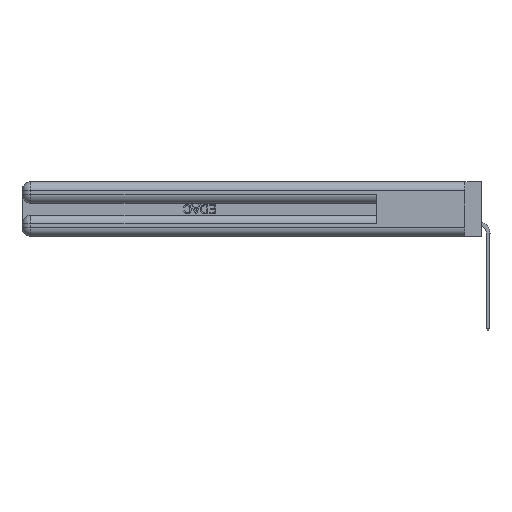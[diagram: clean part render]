
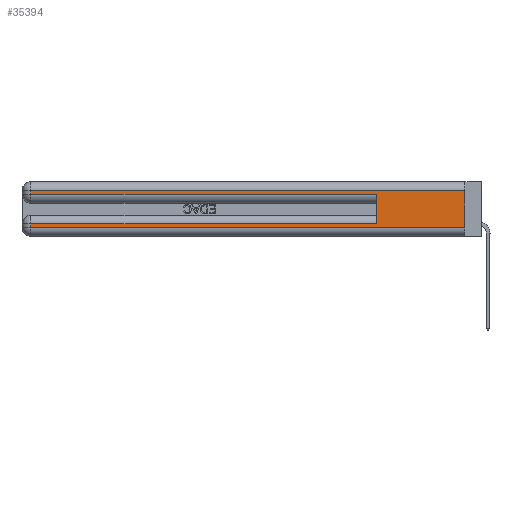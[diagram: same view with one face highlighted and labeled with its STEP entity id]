
A CAD part, left-side view. The second image highlights one B-rep face of the part: STEP entity #35394.
In plain terms, the highlighted planar face has unit normal (-1, 0, 0).
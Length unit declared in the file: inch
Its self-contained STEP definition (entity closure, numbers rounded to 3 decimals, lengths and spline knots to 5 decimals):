
#457 = CARTESIAN_POINT ( 'NONE',  ( 0., 2.94, 0.285 ) ) ;
#775 = EDGE_CURVE ( 'NONE', #44363, #33501, #40268, .T. ) ;
#856 = ORIENTED_EDGE ( 'NONE', *, *, #20694, .T. ) ;
#1387 = CARTESIAN_POINT ( 'NONE',  ( 0., 2.94, 0.37 ) ) ;
#3779 = EDGE_CURVE ( 'NONE', #34875, #40373, #24281, .T. ) ;
#3795 = VECTOR ( 'NONE', #15402, 39.37008 ) ;
#4311 = CARTESIAN_POINT ( 'NONE',  ( 0., 0.6, 0.145 ) ) ;
#4774 = VECTOR ( 'NONE', #35210, 39.37008 ) ;
#5771 = DIRECTION ( 'NONE',  ( 0., -1., 0. ) ) ;
#5900 = CARTESIAN_POINT ( 'NONE',  ( 0., 0., 0.31 ) ) ;
#5971 = DIRECTION ( 'NONE',  ( 0., 0., -1. ) ) ;
#6256 = LINE ( 'NONE', #1387, #13732 ) ;
#6915 = EDGE_CURVE ( 'NONE', #35294, #33501, #15475, .T. ) ;
#9923 = CARTESIAN_POINT ( 'NONE',  ( 0., 2.94, 0.37 ) ) ;
#11583 = ORIENTED_EDGE ( 'NONE', *, *, #41919, .T. ) ;
#12135 = CARTESIAN_POINT ( 'NONE',  ( 0., 0., 0.285 ) ) ;
#13319 = DIRECTION ( 'NONE',  ( 0., 0., -1. ) ) ;
#13518 = EDGE_CURVE ( 'NONE', #40814, #44363, #6256, .T. ) ;
#13732 = VECTOR ( 'NONE', #28822, 39.37008 ) ;
#14787 = DIRECTION ( 'NONE',  ( 0., 0., -1. ) ) ;
#15099 = AXIS2_PLACEMENT_3D ( 'NONE', #43406, #29791, #5971 ) ;
#15130 = VECTOR ( 'NONE', #27407, 39.37008 ) ;
#15402 = DIRECTION ( 'NONE',  ( 0., -1., 0. ) ) ;
#15475 = LINE ( 'NONE', #4311, #4774 ) ;
#16204 = DIRECTION ( 'NONE',  ( 0., 1., 0. ) ) ;
#17505 = CARTESIAN_POINT ( 'NONE',  ( 0., 0., 0.085 ) ) ;
#19222 = FACE_OUTER_BOUND ( 'NONE', #30261, .T. ) ;
#19394 = LINE ( 'NONE', #17505, #15130 ) ;
#20512 = LINE ( 'NONE', #22964, #35559 ) ;
#20694 = EDGE_CURVE ( 'NONE', #34875, #40814, #29694, .T. ) ;
#21058 = CARTESIAN_POINT ( 'NONE',  ( 0., 0., 0.37 ) ) ;
#22111 = VECTOR ( 'NONE', #14787, 39.37008 ) ;
#22132 = LINE ( 'NONE', #9923, #26971 ) ;
#22964 = CARTESIAN_POINT ( 'NONE',  ( 0., 0., 0.06 ) ) ;
#24281 = LINE ( 'NONE', #21058, #22111 ) ;
#26465 = PLANE ( 'NONE',  #15099 ) ;
#26871 = ORIENTED_EDGE ( 'NONE', *, *, #775, .T. ) ;
#26971 = VECTOR ( 'NONE', #13319, 39.37008 ) ;
#27209 = CARTESIAN_POINT ( 'NONE',  ( 0., 0., 0.06 ) ) ;
#27407 = DIRECTION ( 'NONE',  ( 0., 1., 0. ) ) ;
#27806 = CARTESIAN_POINT ( 'NONE',  ( 0., 2.94, 0.085 ) ) ;
#28135 = VERTEX_POINT ( 'NONE', #27806 ) ;
#28822 = DIRECTION ( 'NONE',  ( 0., 0., -1. ) ) ;
#29315 = CARTESIAN_POINT ( 'NONE',  ( 0., 0., 0.31 ) ) ;
#29694 = LINE ( 'NONE', #5900, #34015 ) ;
#29716 = ORIENTED_EDGE ( 'NONE', *, *, #13518, .T. ) ;
#29791 = DIRECTION ( 'NONE',  ( 1., 0., 0. ) ) ;
#30261 = EDGE_LOOP ( 'NONE', ( #31614, #856, #29716, #26871, #39343, #40999, #11583, #32832 ) ) ;
#31614 = ORIENTED_EDGE ( 'NONE', *, *, #3779, .F. ) ;
#32832 = ORIENTED_EDGE ( 'NONE', *, *, #38927, .T. ) ;
#33501 = VERTEX_POINT ( 'NONE', #44139 ) ;
#33591 = CARTESIAN_POINT ( 'NONE',  ( 0., 2.94, 0.31 ) ) ;
#34015 = VECTOR ( 'NONE', #16204, 39.37008 ) ;
#34579 = EDGE_CURVE ( 'NONE', #35294, #28135, #19394, .T. ) ;
#34875 = VERTEX_POINT ( 'NONE', #29315 ) ;
#35210 = DIRECTION ( 'NONE',  ( 0., 0., 1. ) ) ;
#35294 = VERTEX_POINT ( 'NONE', #40410 ) ;
#35394 = ADVANCED_FACE ( 'NONE', ( #19222 ), #26465, .F. ) ;
#35559 = VECTOR ( 'NONE', #5771, 39.37008 ) ;
#36692 = CARTESIAN_POINT ( 'NONE',  ( 0., 2.94, 0.06 ) ) ;
#38927 = EDGE_CURVE ( 'NONE', #43652, #40373, #20512, .T. ) ;
#39343 = ORIENTED_EDGE ( 'NONE', *, *, #6915, .F. ) ;
#40268 = LINE ( 'NONE', #12135, #3795 ) ;
#40373 = VERTEX_POINT ( 'NONE', #27209 ) ;
#40410 = CARTESIAN_POINT ( 'NONE',  ( 0., 0.6, 0.085 ) ) ;
#40814 = VERTEX_POINT ( 'NONE', #33591 ) ;
#40999 = ORIENTED_EDGE ( 'NONE', *, *, #34579, .T. ) ;
#41919 = EDGE_CURVE ( 'NONE', #28135, #43652, #22132, .T. ) ;
#43406 = CARTESIAN_POINT ( 'NONE',  ( 0., 0., 0.37 ) ) ;
#43652 = VERTEX_POINT ( 'NONE', #36692 ) ;
#44139 = CARTESIAN_POINT ( 'NONE',  ( 0., 0.6, 0.285 ) ) ;
#44363 = VERTEX_POINT ( 'NONE', #457 ) ;
